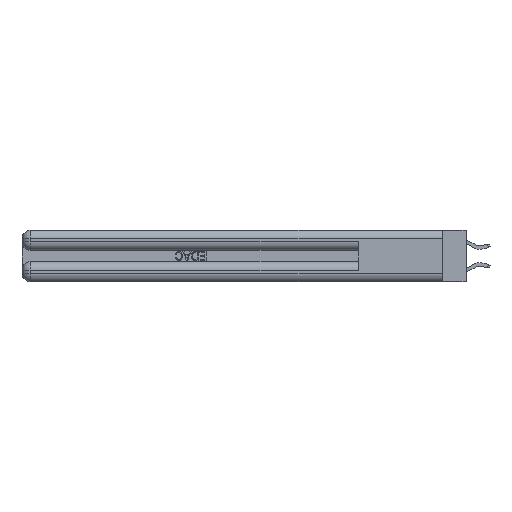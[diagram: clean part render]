
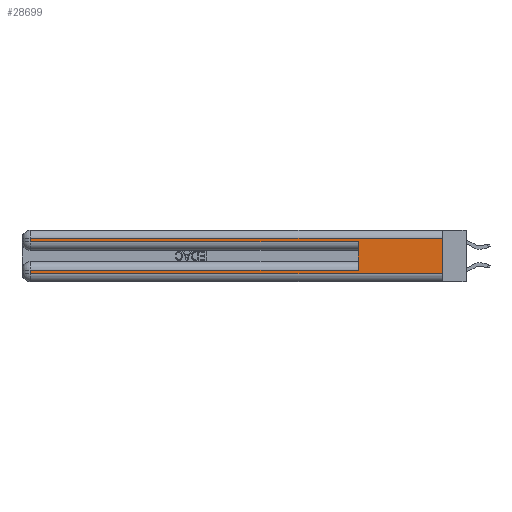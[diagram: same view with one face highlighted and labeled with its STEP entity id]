
A CAD part, left-side view. The second image highlights one B-rep face of the part: STEP entity #28699.
In plain terms, the highlighted planar face has unit normal (-1, 0, 0).
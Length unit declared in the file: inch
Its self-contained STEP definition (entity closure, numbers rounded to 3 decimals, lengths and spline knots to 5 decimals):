
#188 = VERTEX_POINT ( 'NONE', #27556 ) ;
#229 = VECTOR ( 'NONE', #18168, 39.37008 ) ;
#659 = VECTOR ( 'NONE', #11566, 39.37008 ) ;
#1312 = ORIENTED_EDGE ( 'NONE', *, *, #34360, .F. ) ;
#2123 = ORIENTED_EDGE ( 'NONE', *, *, #12574, .T. ) ;
#2554 = LINE ( 'NONE', #23817, #3558 ) ;
#3207 = CARTESIAN_POINT ( 'NONE',  ( 0., 2.94, 0.37 ) ) ;
#3296 = CARTESIAN_POINT ( 'NONE',  ( 0., 0., 0.31 ) ) ;
#3558 = VECTOR ( 'NONE', #10571, 39.37008 ) ;
#3802 = EDGE_CURVE ( 'NONE', #3811, #10599, #22215, .T. ) ;
#3811 = VERTEX_POINT ( 'NONE', #27450 ) ;
#4224 = ORIENTED_EDGE ( 'NONE', *, *, #28603, .F. ) ;
#4736 = VECTOR ( 'NONE', #11323, 39.37008 ) ;
#6158 = DIRECTION ( 'NONE',  ( 0., -1., 0. ) ) ;
#6258 = ORIENTED_EDGE ( 'NONE', *, *, #18726, .T. ) ;
#7262 = CARTESIAN_POINT ( 'NONE',  ( 0., 0.6, 0.085 ) ) ;
#7358 = PLANE ( 'NONE',  #14673 ) ;
#8392 = CARTESIAN_POINT ( 'NONE',  ( 0., 0., 0.06 ) ) ;
#8820 = VECTOR ( 'NONE', #12295, 39.37008 ) ;
#10096 = LINE ( 'NONE', #15488, #22244 ) ;
#10199 = EDGE_CURVE ( 'NONE', #31823, #3811, #15045, .T. ) ;
#10318 = DIRECTION ( 'NONE',  ( 0., 0., -1. ) ) ;
#10571 = DIRECTION ( 'NONE',  ( 0., 0., -1. ) ) ;
#10599 = VERTEX_POINT ( 'NONE', #27935 ) ;
#11218 = CARTESIAN_POINT ( 'NONE',  ( 0., 0., 0.285 ) ) ;
#11323 = DIRECTION ( 'NONE',  ( 0., 1., 0. ) ) ;
#11566 = DIRECTION ( 'NONE',  ( 0., 0., -1. ) ) ;
#11611 = ORIENTED_EDGE ( 'NONE', *, *, #10199, .T. ) ;
#12295 = DIRECTION ( 'NONE',  ( 0., 0., 1. ) ) ;
#12574 = EDGE_CURVE ( 'NONE', #10599, #13614, #10096, .T. ) ;
#12927 = DIRECTION ( 'NONE',  ( 1., 0., 0. ) ) ;
#13187 = EDGE_LOOP ( 'NONE', ( #4224, #20245, #20818, #6258, #1312, #11611, #21689, #2123 ) ) ;
#13614 = VERTEX_POINT ( 'NONE', #8392 ) ;
#14442 = LINE ( 'NONE', #3296, #4736 ) ;
#14673 = AXIS2_PLACEMENT_3D ( 'NONE', #31606, #12927, #10318 ) ;
#15045 = LINE ( 'NONE', #23091, #27181 ) ;
#15488 = CARTESIAN_POINT ( 'NONE',  ( 0., 0., 0.06 ) ) ;
#15955 = VERTEX_POINT ( 'NONE', #24349 ) ;
#16481 = CARTESIAN_POINT ( 'NONE',  ( 0., 0.6, 0.285 ) ) ;
#18168 = DIRECTION ( 'NONE',  ( 0., 0., -1. ) ) ;
#18726 = EDGE_CURVE ( 'NONE', #15955, #32199, #32839, .T. ) ;
#20245 = ORIENTED_EDGE ( 'NONE', *, *, #29874, .T. ) ;
#20604 = CARTESIAN_POINT ( 'NONE',  ( 0., 0., 0.37 ) ) ;
#20818 = ORIENTED_EDGE ( 'NONE', *, *, #21071, .T. ) ;
#21071 = EDGE_CURVE ( 'NONE', #188, #15955, #2554, .T. ) ;
#21120 = LINE ( 'NONE', #20604, #229 ) ;
#21689 = ORIENTED_EDGE ( 'NONE', *, *, #3802, .T. ) ;
#22215 = LINE ( 'NONE', #3207, #659 ) ;
#22244 = VECTOR ( 'NONE', #28932, 39.37008 ) ;
#22776 = CARTESIAN_POINT ( 'NONE',  ( 0., 0.6, 0.145 ) ) ;
#23091 = CARTESIAN_POINT ( 'NONE',  ( 0., 0., 0.085 ) ) ;
#23817 = CARTESIAN_POINT ( 'NONE',  ( 0., 2.94, 0.37 ) ) ;
#24349 = CARTESIAN_POINT ( 'NONE',  ( 0., 2.94, 0.285 ) ) ;
#25552 = LINE ( 'NONE', #22776, #8820 ) ;
#27181 = VECTOR ( 'NONE', #33731, 39.37008 ) ;
#27265 = CARTESIAN_POINT ( 'NONE',  ( 0., 0., 0.31 ) ) ;
#27450 = CARTESIAN_POINT ( 'NONE',  ( 0., 2.94, 0.085 ) ) ;
#27556 = CARTESIAN_POINT ( 'NONE',  ( 0., 2.94, 0.31 ) ) ;
#27935 = CARTESIAN_POINT ( 'NONE',  ( 0., 2.94, 0.06 ) ) ;
#28365 = VERTEX_POINT ( 'NONE', #27265 ) ;
#28603 = EDGE_CURVE ( 'NONE', #28365, #13614, #21120, .T. ) ;
#28699 = ADVANCED_FACE ( 'NONE', ( #33865 ), #7358, .F. ) ;
#28932 = DIRECTION ( 'NONE',  ( 0., -1., 0. ) ) ;
#29874 = EDGE_CURVE ( 'NONE', #28365, #188, #14442, .T. ) ;
#31606 = CARTESIAN_POINT ( 'NONE',  ( 0., 0., 0.37 ) ) ;
#31823 = VERTEX_POINT ( 'NONE', #7262 ) ;
#32199 = VERTEX_POINT ( 'NONE', #16481 ) ;
#32839 = LINE ( 'NONE', #11218, #34163 ) ;
#33731 = DIRECTION ( 'NONE',  ( 0., 1., 0. ) ) ;
#33865 = FACE_OUTER_BOUND ( 'NONE', #13187, .T. ) ;
#34163 = VECTOR ( 'NONE', #6158, 39.37008 ) ;
#34360 = EDGE_CURVE ( 'NONE', #31823, #32199, #25552, .T. ) ;
